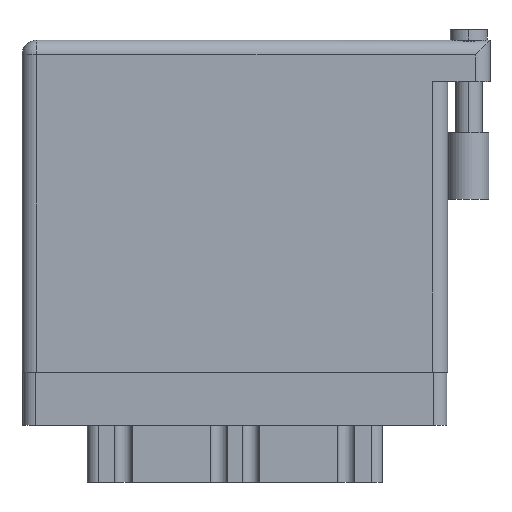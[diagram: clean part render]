
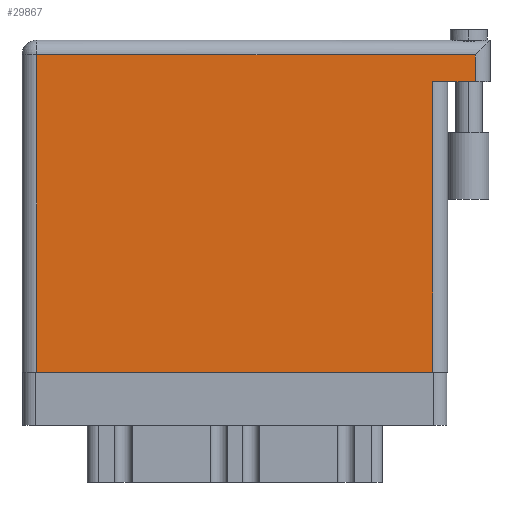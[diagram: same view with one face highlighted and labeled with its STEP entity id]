
A CAD part, front view. The second image highlights one B-rep face of the part: STEP entity #29867.
In plain terms, the highlighted face is planar.
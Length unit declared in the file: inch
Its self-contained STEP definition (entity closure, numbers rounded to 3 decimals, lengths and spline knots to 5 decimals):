
#263 = LINE ( 'NONE', #450, #22865 ) ;
#450 = CARTESIAN_POINT ( 'NONE',  ( 2.208, 1.369, 0. ) ) ;
#797 = CARTESIAN_POINT ( 'NONE',  ( 1.938, 1.369, 0. ) ) ;
#1600 = VERTEX_POINT ( 'NONE', #13402 ) ;
#3469 = VERTEX_POINT ( 'NONE', #33084 ) ;
#5755 = DIRECTION ( 'NONE',  ( -1., 0., 0. ) ) ;
#8052 = FACE_OUTER_BOUND ( 'NONE', #10317, .T. ) ;
#8407 = DIRECTION ( 'NONE',  ( 0., 0., -1. ) ) ;
#8509 = AXIS2_PLACEMENT_3D ( 'NONE', #23897, #8407, #5755 ) ;
#9049 = ORIENTED_EDGE ( 'NONE', *, *, #11767, .T. ) ;
#9185 = EDGE_CURVE ( 'NONE', #3469, #30756, #263, .T. ) ;
#9575 = VERTEX_POINT ( 'NONE', #18875 ) ;
#9908 = VERTEX_POINT ( 'NONE', #18989 ) ;
#10114 = VERTEX_POINT ( 'NONE', #12739 ) ;
#10317 = EDGE_LOOP ( 'NONE', ( #24679, #31710, #14603, #17770, #24950, #9049 ) ) ;
#10404 = VECTOR ( 'NONE', #27688, 39.37008 ) ;
#11101 = DIRECTION ( 'NONE',  ( -1., 0., 0. ) ) ;
#11530 = EDGE_CURVE ( 'NONE', #1600, #9575, #19678, .T. ) ;
#11767 = EDGE_CURVE ( 'NONE', #9575, #9908, #13566, .T. ) ;
#12549 = DIRECTION ( 'NONE',  ( -1., 0., 0. ) ) ;
#12739 = CARTESIAN_POINT ( 'NONE',  ( 1.938, 0., 0. ) ) ;
#13402 = CARTESIAN_POINT ( 'NONE',  ( 2.138, 1.496, 0. ) ) ;
#13566 = LINE ( 'NONE', #29263, #14670 ) ;
#14078 = CARTESIAN_POINT ( 'NONE',  ( 0., 0., 0. ) ) ;
#14603 = ORIENTED_EDGE ( 'NONE', *, *, #9185, .F. ) ;
#14670 = VECTOR ( 'NONE', #21397, 39.37008 ) ;
#15449 = EDGE_CURVE ( 'NONE', #3469, #1600, #31614, .T. ) ;
#16967 = DIRECTION ( 'NONE',  ( 0., 1., 0. ) ) ;
#17770 = ORIENTED_EDGE ( 'NONE', *, *, #15449, .T. ) ;
#18334 = PLANE ( 'NONE',  #8509 ) ;
#18837 = DIRECTION ( 'NONE',  ( 0., 1., 0. ) ) ;
#18875 = CARTESIAN_POINT ( 'NONE',  ( 0.07, 1.496, 0. ) ) ;
#18989 = CARTESIAN_POINT ( 'NONE',  ( 0.07, 0., 0. ) ) ;
#19678 = LINE ( 'NONE', #22825, #20954 ) ;
#20954 = VECTOR ( 'NONE', #12549, 39.37008 ) ;
#21397 = DIRECTION ( 'NONE',  ( 0., -1., 0. ) ) ;
#22825 = CARTESIAN_POINT ( 'NONE',  ( 0., 1.496, 0. ) ) ;
#22865 = VECTOR ( 'NONE', #11101, 39.37008 ) ;
#23268 = LINE ( 'NONE', #14078, #10404 ) ;
#23897 = CARTESIAN_POINT ( 'NONE',  ( 0., 1.566, 0. ) ) ;
#24029 = CARTESIAN_POINT ( 'NONE',  ( 2.138, 1.566, 0. ) ) ;
#24191 = VECTOR ( 'NONE', #16967, 39.37008 ) ;
#24679 = ORIENTED_EDGE ( 'NONE', *, *, #33500, .T. ) ;
#24950 = ORIENTED_EDGE ( 'NONE', *, *, #11530, .T. ) ;
#24995 = CARTESIAN_POINT ( 'NONE',  ( 1.938, 1.369, 0. ) ) ;
#27103 = EDGE_CURVE ( 'NONE', #10114, #30756, #32517, .T. ) ;
#27600 = VECTOR ( 'NONE', #18837, 39.37008 ) ;
#27688 = DIRECTION ( 'NONE',  ( 1., 0., 0. ) ) ;
#29263 = CARTESIAN_POINT ( 'NONE',  ( 0.07, 0., 0. ) ) ;
#29867 = ADVANCED_FACE ( 'NONE', ( #8052 ), #18334, .F. ) ;
#30756 = VERTEX_POINT ( 'NONE', #797 ) ;
#31614 = LINE ( 'NONE', #24029, #27600 ) ;
#31710 = ORIENTED_EDGE ( 'NONE', *, *, #27103, .T. ) ;
#32517 = LINE ( 'NONE', #24995, #24191 ) ;
#33084 = CARTESIAN_POINT ( 'NONE',  ( 2.138, 1.369, 0. ) ) ;
#33500 = EDGE_CURVE ( 'NONE', #9908, #10114, #23268, .T. ) ;
